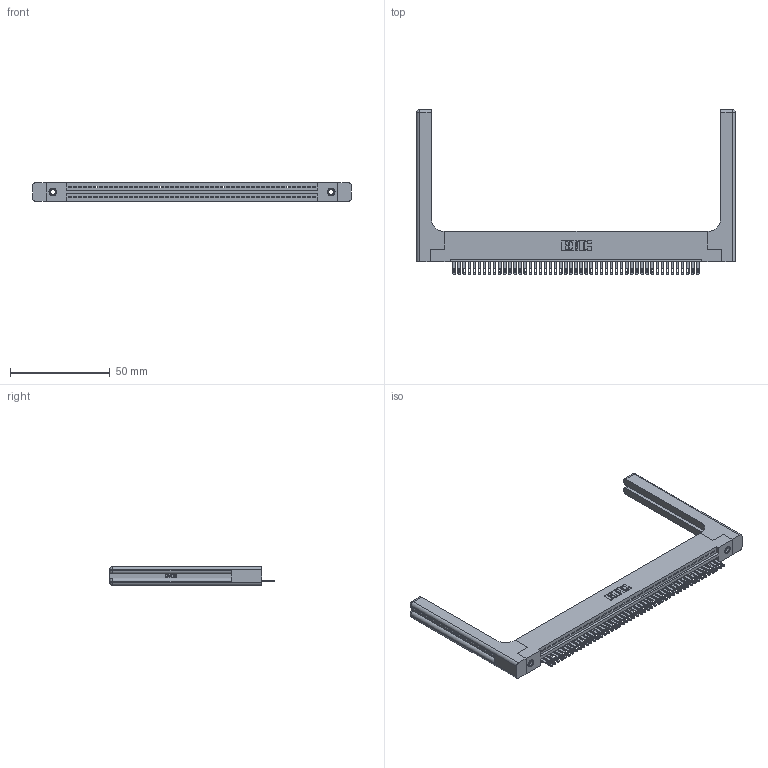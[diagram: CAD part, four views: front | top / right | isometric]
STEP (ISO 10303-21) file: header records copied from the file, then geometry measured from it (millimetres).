
FILE_DESCRIPTION (( 'STEP AP203' ), '1' );
FILE_NAME ('345-049-500-158.STEP', '2019-10-09T06:52:53', ( '' ), ( '' ), 'SwSTEP 2.0', 'SolidWorks 2016', '' );
FILE_SCHEMA (( 'CONFIG_CONTROL_DESIGN' ));
Length unit declared in the file: inch
Products named in the file (5): 345-292-001_345-293-100; 345-250-001_345-250-001-102; 345-049-500-158; 345-220-058_345-220-058; 345 Part_Flush Mounting Lugs - 0.156 Dia-TH
Assembly tree (54 placements, depth 2):
  345-049-500-158
    345 Part_Flush Mounting Lugs - 0.156 Dia-TH
    345-292-001_345-293-100  x49
    345-250-001_345-250-001-102  x2
    345-220-058_345-220-058  x2
Bounding box: 159.49 x 82.47 x 9.4 mm (x, y, z)
Volume: 23740.8 mm3; surface area: 25757.8 mm2
Topology: 54 solids, 54 shells, 3028 faces, 9239 edges, 6138 vertices
Faces by surface type: plane 1894, cylinder 1074, bspline 36, cone 12, sphere 8, torus 4
Entity records: 41048 total; most frequent: CARTESIAN_POINT 8080, ORIENTED_EDGE 6860, DIRECTION 5996, EDGE_CURVE 3430, LINE 3006, VECTOR 3006, VERTEX_POINT 2278, AXIS2_PLACEMENT_3D 1495
